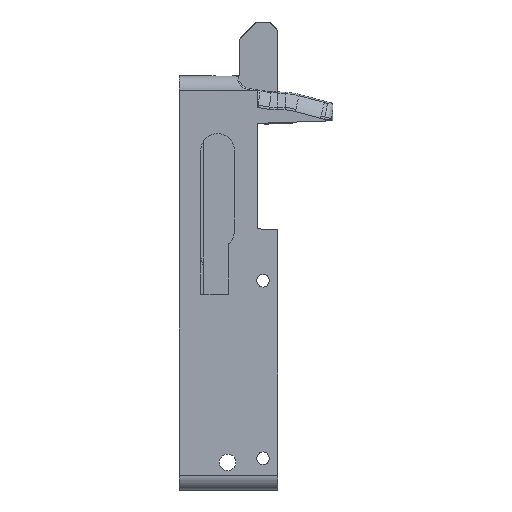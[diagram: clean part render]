
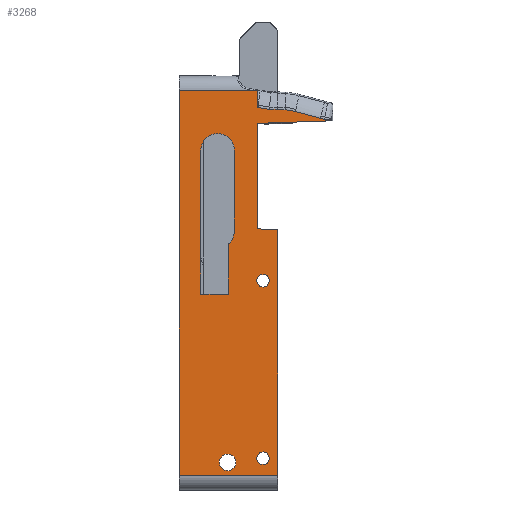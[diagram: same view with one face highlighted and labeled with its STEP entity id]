
A CAD part, left-side view. The second image highlights one B-rep face of the part: STEP entity #3268.
In plain terms, the highlighted planar face has unit normal (-1, 0, 0).
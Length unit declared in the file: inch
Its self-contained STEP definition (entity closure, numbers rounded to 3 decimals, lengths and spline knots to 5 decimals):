
#41=FACE_BOUND('',#921,.T.);
#42=FACE_BOUND('',#922,.T.);
#43=FACE_BOUND('',#923,.T.);
#44=FACE_BOUND('',#924,.T.);
#77=PLANE('',#3476);
#152=LINE('',#4819,#412);
#153=LINE('',#4822,#413);
#154=LINE('',#4824,#414);
#155=LINE('',#4826,#415);
#156=LINE('',#4828,#416);
#157=LINE('',#4830,#417);
#158=LINE('',#4832,#418);
#159=LINE('',#4834,#419);
#160=LINE('',#4836,#420);
#161=LINE('',#4838,#421);
#162=LINE('',#4840,#422);
#163=LINE('',#4847,#423);
#164=LINE('',#4849,#424);
#165=LINE('',#4851,#425);
#166=LINE('',#4853,#426);
#167=LINE('',#4854,#427);
#168=LINE('',#4859,#428);
#169=LINE('',#4861,#429);
#170=LINE('',#4863,#430);
#171=LINE('',#4867,#431);
#412=VECTOR('',#3803,0.02);
#413=VECTOR('',#3806,0.3937);
#414=VECTOR('',#3807,0.3937);
#415=VECTOR('',#3808,0.3937);
#416=VECTOR('',#3809,0.3937);
#417=VECTOR('',#3810,0.3937);
#418=VECTOR('',#3811,0.3937);
#419=VECTOR('',#3812,0.3937);
#420=VECTOR('',#3813,0.3937);
#421=VECTOR('',#3814,0.3937);
#422=VECTOR('',#3815,0.3937);
#423=VECTOR('',#3816,0.3937);
#424=VECTOR('',#3817,0.3937);
#425=VECTOR('',#3818,0.3937);
#426=VECTOR('',#3819,0.3937);
#427=VECTOR('',#3820,0.3937);
#428=VECTOR('',#3823,0.3937);
#429=VECTOR('',#3824,0.3937);
#430=VECTOR('',#3825,0.3937);
#431=VECTOR('',#3828,0.3937);
#736=FACE_OUTER_BOUND('',#920,.T.);
#920=EDGE_LOOP('',(#2239,#2240,#2241,#2242,#2243,#2244,#2245,#2246,#2247,
#2248,#2249,#2250,#2251,#2252,#2253,#2254,#2255));
#921=EDGE_LOOP('',(#2256,#2257,#2258,#2259,#2260,#2261,#2262));
#922=EDGE_LOOP('',(#2263));
#923=EDGE_LOOP('',(#2264));
#924=EDGE_LOOP('',(#2265));
#1138=CIRCLE('',#3477,0.1);
#1139=CIRCLE('',#3478,0.25);
#1140=CIRCLE('',#3479,0.25);
#1141=CIRCLE('',#3480,0.125);
#1142=CIRCLE('',#3481,0.094);
#1143=CIRCLE('',#3482,0.094);
#1316=B_SPLINE_CURVE_WITH_KNOTS('',3,(#4842,#4843,#4844,#4845),
 .UNSPECIFIED.,.F.,.F.,(4,4),(-0.39206,0.00034),
 .UNSPECIFIED.);
#1387=VERTEX_POINT('',#4720);
#1391=VERTEX_POINT('',#4815);
#1393=VERTEX_POINT('',#4821);
#1394=VERTEX_POINT('',#4823);
#1395=VERTEX_POINT('',#4825);
#1396=VERTEX_POINT('',#4827);
#1397=VERTEX_POINT('',#4829);
#1398=VERTEX_POINT('',#4831);
#1399=VERTEX_POINT('',#4833);
#1400=VERTEX_POINT('',#4835);
#1401=VERTEX_POINT('',#4837);
#1402=VERTEX_POINT('',#4839);
#1403=VERTEX_POINT('',#4841);
#1404=VERTEX_POINT('',#4846);
#1405=VERTEX_POINT('',#4848);
#1406=VERTEX_POINT('',#4850);
#1407=VERTEX_POINT('',#4852);
#1408=VERTEX_POINT('',#4855);
#1409=VERTEX_POINT('',#4856);
#1410=VERTEX_POINT('',#4858);
#1411=VERTEX_POINT('',#4860);
#1412=VERTEX_POINT('',#4862);
#1413=VERTEX_POINT('',#4864);
#1414=VERTEX_POINT('',#4866);
#1415=VERTEX_POINT('',#4869);
#1416=VERTEX_POINT('',#4871);
#1417=VERTEX_POINT('',#4873);
#1728=EDGE_CURVE('',#1387,#1391,#152,.T.);
#1729=EDGE_CURVE('',#1387,#1393,#153,.T.);
#1730=EDGE_CURVE('',#1394,#1393,#154,.T.);
#1731=EDGE_CURVE('',#1395,#1394,#155,.T.);
#1732=EDGE_CURVE('',#1395,#1396,#156,.T.);
#1733=EDGE_CURVE('',#1396,#1397,#157,.T.);
#1734=EDGE_CURVE('',#1397,#1398,#158,.T.);
#1735=EDGE_CURVE('',#1398,#1399,#159,.T.);
#1736=EDGE_CURVE('',#1400,#1399,#160,.T.);
#1737=EDGE_CURVE('',#1401,#1400,#161,.T.);
#1738=EDGE_CURVE('',#1402,#1401,#162,.T.);
#1739=EDGE_CURVE('',#1403,#1402,#1316,.T.);
#1740=EDGE_CURVE('',#1404,#1403,#163,.T.);
#1741=EDGE_CURVE('',#1405,#1404,#164,.T.);
#1742=EDGE_CURVE('',#1406,#1405,#165,.T.);
#1743=EDGE_CURVE('',#1406,#1407,#166,.T.);
#1744=EDGE_CURVE('',#1407,#1391,#167,.T.);
#1745=EDGE_CURVE('',#1408,#1409,#1138,.T.);
#1746=EDGE_CURVE('',#1408,#1410,#168,.T.);
#1747=EDGE_CURVE('',#1410,#1411,#169,.T.);
#1748=EDGE_CURVE('',#1411,#1412,#170,.T.);
#1749=EDGE_CURVE('',#1412,#1413,#1139,.T.);
#1750=EDGE_CURVE('',#1413,#1414,#171,.T.);
#1751=EDGE_CURVE('',#1414,#1409,#1140,.T.);
#1752=EDGE_CURVE('',#1415,#1415,#1141,.T.);
#1753=EDGE_CURVE('',#1416,#1416,#1142,.T.);
#1754=EDGE_CURVE('',#1417,#1417,#1143,.T.);
#2239=ORIENTED_EDGE('',*,*,#1728,.F.);
#2240=ORIENTED_EDGE('',*,*,#1729,.T.);
#2241=ORIENTED_EDGE('',*,*,#1730,.F.);
#2242=ORIENTED_EDGE('',*,*,#1731,.F.);
#2243=ORIENTED_EDGE('',*,*,#1732,.T.);
#2244=ORIENTED_EDGE('',*,*,#1733,.T.);
#2245=ORIENTED_EDGE('',*,*,#1734,.T.);
#2246=ORIENTED_EDGE('',*,*,#1735,.T.);
#2247=ORIENTED_EDGE('',*,*,#1736,.F.);
#2248=ORIENTED_EDGE('',*,*,#1737,.F.);
#2249=ORIENTED_EDGE('',*,*,#1738,.F.);
#2250=ORIENTED_EDGE('',*,*,#1739,.F.);
#2251=ORIENTED_EDGE('',*,*,#1740,.F.);
#2252=ORIENTED_EDGE('',*,*,#1741,.F.);
#2253=ORIENTED_EDGE('',*,*,#1742,.F.);
#2254=ORIENTED_EDGE('',*,*,#1743,.T.);
#2255=ORIENTED_EDGE('',*,*,#1744,.T.);
#2256=ORIENTED_EDGE('',*,*,#1745,.F.);
#2257=ORIENTED_EDGE('',*,*,#1746,.T.);
#2258=ORIENTED_EDGE('',*,*,#1747,.T.);
#2259=ORIENTED_EDGE('',*,*,#1748,.T.);
#2260=ORIENTED_EDGE('',*,*,#1749,.T.);
#2261=ORIENTED_EDGE('',*,*,#1750,.T.);
#2262=ORIENTED_EDGE('',*,*,#1751,.T.);
#2263=ORIENTED_EDGE('',*,*,#1752,.T.);
#2264=ORIENTED_EDGE('',*,*,#1753,.T.);
#2265=ORIENTED_EDGE('',*,*,#1754,.T.);
#3268=ADVANCED_FACE('',(#736,#41,#42,#43,#44),#77,.T.);
#3476=AXIS2_PLACEMENT_3D('',#4820,#3804,#3805);
#3477=AXIS2_PLACEMENT_3D('',#4857,#3821,#3822);
#3478=AXIS2_PLACEMENT_3D('',#4865,#3826,#3827);
#3479=AXIS2_PLACEMENT_3D('',#4868,#3829,#3830);
#3480=AXIS2_PLACEMENT_3D('',#4870,#3831,#3832);
#3481=AXIS2_PLACEMENT_3D('',#4872,#3833,#3834);
#3482=AXIS2_PLACEMENT_3D('',#4874,#3835,#3836);
#3803=DIRECTION('',(0.,-0.988,-0.151));
#3804=DIRECTION('center_axis',(-1.,0.,0.));
#3805=DIRECTION('ref_axis',(0.,0.,1.));
#3806=DIRECTION('',(0.,1.,0.));
#3807=DIRECTION('',(0.,0.,1.));
#3808=DIRECTION('',(0.,1.,0.));
#3809=DIRECTION('',(0.,0.,1.));
#3810=DIRECTION('',(0.,0.999,0.035));
#3811=DIRECTION('',(0.,0.,1.));
#3812=DIRECTION('',(0.,-0.999,0.035));
#3813=DIRECTION('',(0.,0.,-1.));
#3814=DIRECTION('',(0.,-0.972,-0.233));
#3815=DIRECTION('',(0.,-0.966,-0.259));
#3816=DIRECTION('',(0.,-0.999,-0.052));
#3817=DIRECTION('',(0.,-1.,0.));
#3818=DIRECTION('',(0.,-0.988,-0.151));
#3819=DIRECTION('',(0.,0.995,0.099));
#3820=DIRECTION('',(0.,0.,1.));
#3821=DIRECTION('center_axis',(1.,0.,0.));
#3822=DIRECTION('ref_axis',(0.,0.934,0.359));
#3823=DIRECTION('',(0.,0.,-1.));
#3824=DIRECTION('',(0.,1.,0.));
#3825=DIRECTION('',(0.,0.,1.));
#3826=DIRECTION('center_axis',(1.,0.,0.));
#3827=DIRECTION('ref_axis',(0.,1.,0.));
#3828=DIRECTION('',(0.,0.,-1.));
#3829=DIRECTION('center_axis',(1.,0.,0.));
#3830=DIRECTION('ref_axis',(0.,-1.,0.));
#3831=DIRECTION('center_axis',(1.,0.,0.));
#3832=DIRECTION('ref_axis',(0.,0.,-1.));
#3833=DIRECTION('center_axis',(1.,0.,0.));
#3834=DIRECTION('ref_axis',(0.,0.,-1.));
#3835=DIRECTION('center_axis',(1.,0.,0.));
#3836=DIRECTION('ref_axis',(0.,0.,-1.));
#4720=CARTESIAN_POINT('',(0.,1.21678,-1.025));
#4815=CARTESIAN_POINT('',(0.,1.1565,-1.03423));
#4819=CARTESIAN_POINT('',(0.,-0.86612,-1.34396));
#4820=CARTESIAN_POINT('Origin',(0.,0.,-7.));
#4821=CARTESIAN_POINT('',(0.,2.325,-1.025));
#4822=CARTESIAN_POINT('',(0.,1.42866,-1.025));
#4823=CARTESIAN_POINT('',(0.,2.325,-6.78));
#4824=CARTESIAN_POINT('',(0.,2.325,-7.));
#4825=CARTESIAN_POINT('',(0.,0.85,-6.78));
#4826=CARTESIAN_POINT('',(0.,0.,-6.78));
#4827=CARTESIAN_POINT('',(0.,0.85,-3.10499));
#4828=CARTESIAN_POINT('',(0.,0.85,-5.0625));
#4829=CARTESIAN_POINT('',(0.,1.1565,-3.09428));
#4830=CARTESIAN_POINT('',(0.,0.35724,-3.1222));
#4831=CARTESIAN_POINT('',(0.,1.1565,-1.51637));
#4832=CARTESIAN_POINT('',(0.,1.1565,-3.15463));
#4833=CARTESIAN_POINT('',(0.,0.14881,-1.48118));
#4834=CARTESIAN_POINT('',(0.,0.68375,-1.49986));
#4835=CARTESIAN_POINT('',(0.,0.14881,-1.45494));
#4836=CARTESIAN_POINT('',(0.,0.14881,-7.));
#4837=CARTESIAN_POINT('',(0.,0.21053,-1.44012));
#4838=CARTESIAN_POINT('',(0.,0.21008,-1.44023));
#4839=CARTESIAN_POINT('',(0.,0.58866,-1.3388));
#4840=CARTESIAN_POINT('',(0.,0.58438,-1.33995));
#4841=CARTESIAN_POINT('',(0.,0.74077,-1.31348));
#4842=CARTESIAN_POINT('Ctrl Pts',(0.,0.74077,
-1.31348));
#4843=CARTESIAN_POINT('Ctrl Pts',(0.,0.68937,
-1.31658));
#4844=CARTESIAN_POINT('Ctrl Pts',(0.,0.63829,
-1.32508));
#4845=CARTESIAN_POINT('Ctrl Pts',(0.,0.58866,
-1.3388));
#4846=CARTESIAN_POINT('',(0.,0.85687,-1.30739));
#4847=CARTESIAN_POINT('',(0.,0.8535,-1.30757));
#4848=CARTESIAN_POINT('',(0.,0.97402,-1.30739));
#4849=CARTESIAN_POINT('',(0.,0.98384,-1.30739));
#4850=CARTESIAN_POINT('',(0.,1.14343,-1.28145));
#4851=CARTESIAN_POINT('',(0.,1.13675,-1.28248));
#4852=CARTESIAN_POINT('',(0.,1.1565,-1.28015));
#4853=CARTESIAN_POINT('',(0.,1.14343,-1.28145));
#4854=CARTESIAN_POINT('',(0.,1.1565,-4.07406));
#4855=CARTESIAN_POINT('',(0.,1.59,-3.36221));
#4856=CARTESIAN_POINT('',(0.,1.56429,-3.29527));
#4857=CARTESIAN_POINT('Origin',(0.,1.49,-3.36221));
#4858=CARTESIAN_POINT('',(0.,1.59,-4.07));
#4859=CARTESIAN_POINT('',(0.,1.59,-5.535));
#4860=CARTESIAN_POINT('',(0.,2.,-4.07));
#4861=CARTESIAN_POINT('',(0.,1.,-4.07));
#4862=CARTESIAN_POINT('',(0.,2.,-1.92));
#4863=CARTESIAN_POINT('',(0.,2.,-4.46));
#4864=CARTESIAN_POINT('',(0.,1.5,-1.92));
#4865=CARTESIAN_POINT('Origin',(0.,1.75,-1.92));
#4866=CARTESIAN_POINT('',(0.,1.5,-3.12791));
#4867=CARTESIAN_POINT('',(0.,1.5,-5.06395));
#4868=CARTESIAN_POINT('Origin',(0.,1.75,-3.12791));
#4869=CARTESIAN_POINT('',(0.,1.6,-6.462));
#4870=CARTESIAN_POINT('Origin',(0.,1.6,-6.587));
#4871=CARTESIAN_POINT('',(0.,1.07,-6.431));
#4872=CARTESIAN_POINT('Origin',(0.,1.07,-6.525));
#4873=CARTESIAN_POINT('',(0.,1.07,-3.776));
#4874=CARTESIAN_POINT('Origin',(0.,1.07,-3.87));
